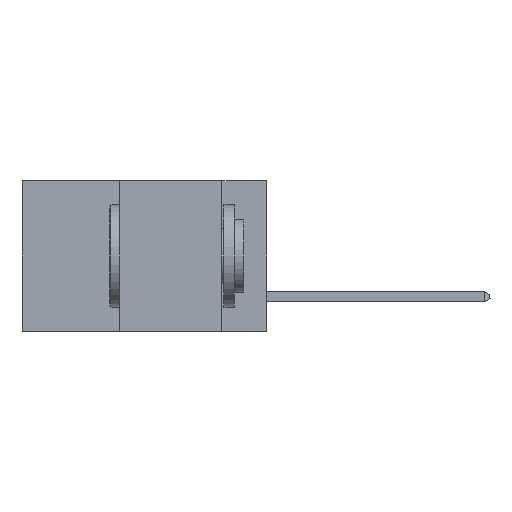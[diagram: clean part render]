
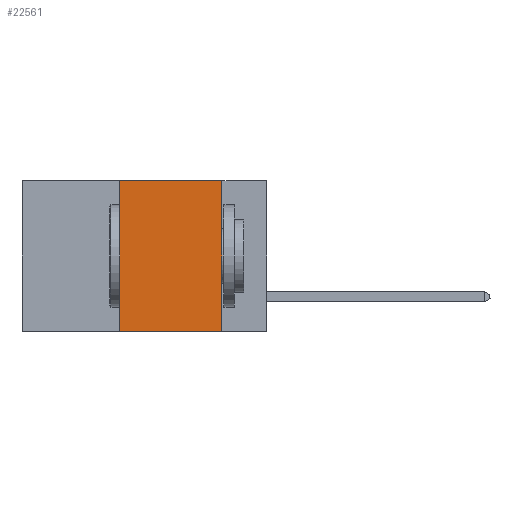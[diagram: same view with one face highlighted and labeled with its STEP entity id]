
A CAD part, left-side view. The second image highlights one B-rep face of the part: STEP entity #22561.
In plain terms, the highlighted planar face has unit normal (-1, 0, 0).
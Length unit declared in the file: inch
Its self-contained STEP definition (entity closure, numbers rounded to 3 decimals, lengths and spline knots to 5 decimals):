
#3769 = VECTOR ( 'NONE', #48856, 39.37008 ) ;
#5453 = DIRECTION ( 'NONE',  ( 0., -1., 0. ) ) ;
#6118 = CARTESIAN_POINT ( 'NONE',  ( 0., 0.6, -0.37 ) ) ;
#6500 = CARTESIAN_POINT ( 'NONE',  ( 0., 0.6, 0. ) ) ;
#7473 = CARTESIAN_POINT ( 'NONE',  ( 0., 0.11, 0. ) ) ;
#7641 = VERTEX_POINT ( 'NONE', #31247 ) ;
#9939 = VERTEX_POINT ( 'NONE', #42777 ) ;
#11968 = EDGE_CURVE ( 'NONE', #25681, #7641, #45681, .T. ) ;
#12164 = CARTESIAN_POINT ( 'NONE',  ( 0., 0.36, 0. ) ) ;
#13009 = LINE ( 'NONE', #37004, #3769 ) ;
#13041 = VECTOR ( 'NONE', #25873, 39.37008 ) ;
#18544 = EDGE_CURVE ( 'NONE', #25681, #9939, #45211, .T. ) ;
#18645 = ORIENTED_EDGE ( 'NONE', *, *, #44979, .F. ) ;
#21630 = AXIS2_PLACEMENT_3D ( 'NONE', #6500, #30375, #42328 ) ;
#22561 = ADVANCED_FACE ( 'NONE', ( #50951 ), #33829, .F. ) ;
#23684 = DIRECTION ( 'NONE',  ( 0., 0., 1. ) ) ;
#24097 = ORIENTED_EDGE ( 'NONE', *, *, #11968, .T. ) ;
#24260 = VECTOR ( 'NONE', #23684, 39.37008 ) ;
#25681 = VERTEX_POINT ( 'NONE', #36464 ) ;
#25873 = DIRECTION ( 'NONE',  ( 0., -1., 0. ) ) ;
#30375 = DIRECTION ( 'NONE',  ( 1., 0., 0. ) ) ;
#30517 = EDGE_LOOP ( 'NONE', ( #43377, #18645, #46990, #24097 ) ) ;
#30918 = VECTOR ( 'NONE', #5453, 39.37008 ) ;
#31247 = CARTESIAN_POINT ( 'NONE',  ( 0., 0.11, -0.37 ) ) ;
#33829 = PLANE ( 'NONE',  #21630 ) ;
#34114 = EDGE_CURVE ( 'NONE', #46485, #7641, #13009, .T. ) ;
#36464 = CARTESIAN_POINT ( 'NONE',  ( 0., 0.36, -0.37 ) ) ;
#37004 = CARTESIAN_POINT ( 'NONE',  ( 0., 0.11, 0. ) ) ;
#41084 = CARTESIAN_POINT ( 'NONE',  ( 0., 0.6, 0. ) ) ;
#41444 = LINE ( 'NONE', #41084, #30918 ) ;
#42328 = DIRECTION ( 'NONE',  ( 0., 0., -1. ) ) ;
#42777 = CARTESIAN_POINT ( 'NONE',  ( 0., 0.36, 0. ) ) ;
#43377 = ORIENTED_EDGE ( 'NONE', *, *, #34114, .F. ) ;
#44979 = EDGE_CURVE ( 'NONE', #9939, #46485, #41444, .T. ) ;
#45211 = LINE ( 'NONE', #12164, #24260 ) ;
#45681 = LINE ( 'NONE', #6118, #13041 ) ;
#46485 = VERTEX_POINT ( 'NONE', #7473 ) ;
#46990 = ORIENTED_EDGE ( 'NONE', *, *, #18544, .F. ) ;
#48856 = DIRECTION ( 'NONE',  ( 0., 0., -1. ) ) ;
#50951 = FACE_OUTER_BOUND ( 'NONE', #30517, .T. ) ;
